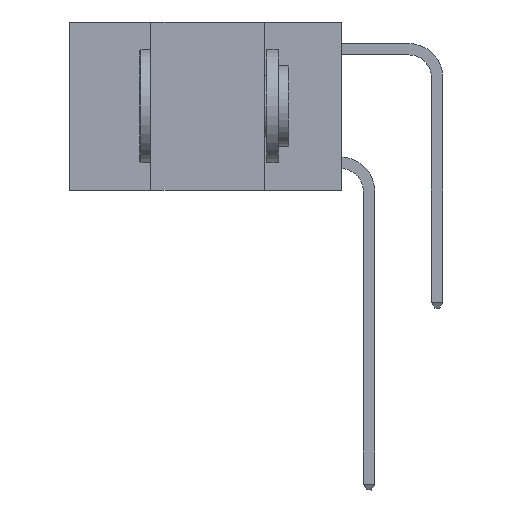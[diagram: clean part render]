
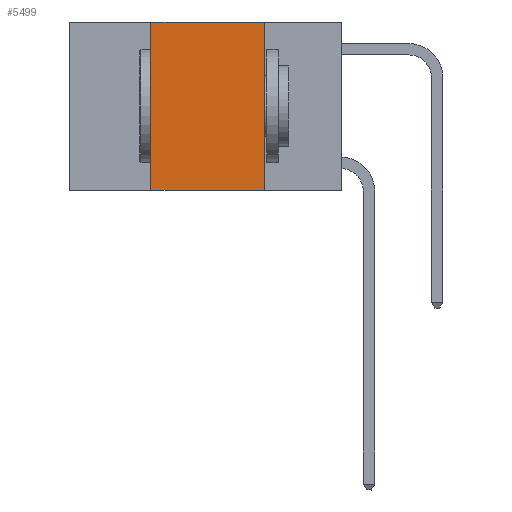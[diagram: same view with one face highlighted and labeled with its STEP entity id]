
A CAD part, left-side view. The second image highlights one B-rep face of the part: STEP entity #5499.
In plain terms, the highlighted planar face has unit normal (-1, 0, 0).
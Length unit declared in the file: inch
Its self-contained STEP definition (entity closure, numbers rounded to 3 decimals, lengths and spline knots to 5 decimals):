
#163 = EDGE_CURVE ( 'NONE', #8165, #13390, #13351, .T. ) ;
#578 = CARTESIAN_POINT ( 'NONE',  ( 0., 0.42, -0.37 ) ) ;
#1268 = CARTESIAN_POINT ( 'NONE',  ( 0., 0.42, 0. ) ) ;
#3218 = ORIENTED_EDGE ( 'NONE', *, *, #7229, .F. ) ;
#3441 = PLANE ( 'NONE',  #3518 ) ;
#3460 = CARTESIAN_POINT ( 'NONE',  ( 0., 0.42, 0. ) ) ;
#3507 = DIRECTION ( 'NONE',  ( 0., 0., 1. ) ) ;
#3518 = AXIS2_PLACEMENT_3D ( 'NONE', #8673, #15828, #5235 ) ;
#3768 = ORIENTED_EDGE ( 'NONE', *, *, #163, .F. ) ;
#3909 = CARTESIAN_POINT ( 'NONE',  ( 0., 0.17, 0. ) ) ;
#5235 = DIRECTION ( 'NONE',  ( 0., 0., -1. ) ) ;
#5499 = ADVANCED_FACE ( 'NONE', ( #17752 ), #3441, .F. ) ;
#5744 = DIRECTION ( 'NONE',  ( 0., 0., -1. ) ) ;
#6474 = DIRECTION ( 'NONE',  ( 0., -1., 0. ) ) ;
#7229 = EDGE_CURVE ( 'NONE', #13390, #10087, #20930, .T. ) ;
#7418 = LINE ( 'NONE', #3909, #16275 ) ;
#7596 = EDGE_CURVE ( 'NONE', #10087, #13683, #7418, .T. ) ;
#7694 = CARTESIAN_POINT ( 'NONE',  ( 0., 0.17, 0. ) ) ;
#8165 = VERTEX_POINT ( 'NONE', #578 ) ;
#8673 = CARTESIAN_POINT ( 'NONE',  ( 0., 0.6, 0. ) ) ;
#9037 = CARTESIAN_POINT ( 'NONE',  ( 0., 0.17, -0.37 ) ) ;
#9944 = EDGE_LOOP ( 'NONE', ( #16780, #3218, #3768, #13170 ) ) ;
#10087 = VERTEX_POINT ( 'NONE', #7694 ) ;
#13170 = ORIENTED_EDGE ( 'NONE', *, *, #20694, .T. ) ;
#13351 = LINE ( 'NONE', #3460, #22091 ) ;
#13390 = VERTEX_POINT ( 'NONE', #1268 ) ;
#13683 = VERTEX_POINT ( 'NONE', #9037 ) ;
#14315 = CARTESIAN_POINT ( 'NONE',  ( 0., 0.6, -0.37 ) ) ;
#15828 = DIRECTION ( 'NONE',  ( 1., 0., 0. ) ) ;
#16275 = VECTOR ( 'NONE', #5744, 39.37008 ) ;
#16780 = ORIENTED_EDGE ( 'NONE', *, *, #7596, .F. ) ;
#17752 = FACE_OUTER_BOUND ( 'NONE', #9944, .T. ) ;
#18802 = CARTESIAN_POINT ( 'NONE',  ( 0., 0.6, 0. ) ) ;
#20392 = VECTOR ( 'NONE', #6474, 39.37008 ) ;
#20663 = LINE ( 'NONE', #14315, #22268 ) ;
#20694 = EDGE_CURVE ( 'NONE', #8165, #13683, #20663, .T. ) ;
#20930 = LINE ( 'NONE', #18802, #20392 ) ;
#21328 = DIRECTION ( 'NONE',  ( 0., -1., 0. ) ) ;
#22091 = VECTOR ( 'NONE', #3507, 39.37008 ) ;
#22268 = VECTOR ( 'NONE', #21328, 39.37008 ) ;
